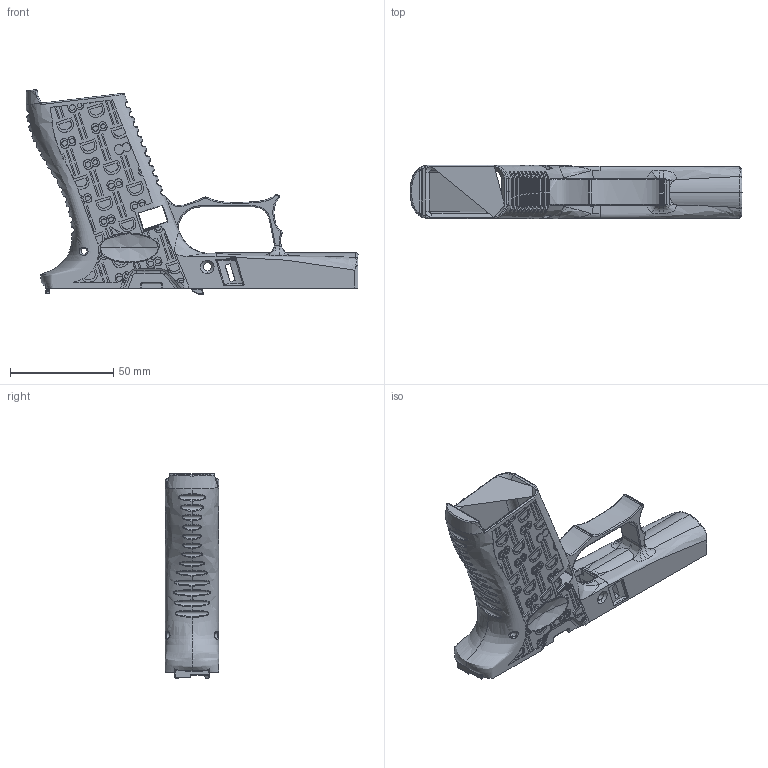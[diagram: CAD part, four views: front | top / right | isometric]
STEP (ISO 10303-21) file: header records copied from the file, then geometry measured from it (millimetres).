
FILE_DESCRIPTION (( 'STEP AP203' ), '1' );
FILE_NAME ('E43X DickinAround SLA.STEP', '2020-12-17T01:37:16', ( '' ), ( '' ), 'SwSTEP 2.0', 'SolidWorks 2016', '' );
FILE_SCHEMA (( 'CONFIG_CONTROL_DESIGN' ));
Products named in the file (1): E43X DickinAround SLA
Bounding box: 160.56 x 25.9 x 98.92 mm (x, y, z)
Volume: 61684.6 mm3; surface area: 39840.1 mm2
Topology: 1 solids, 1 shells, 2598 faces, 6892 edges, 4410 vertices
Faces by surface type: bspline 1189, plane 930, cylinder 433, torus 30, cone 12, sphere 4
Entity records: 383233 total; most frequent: CARTESIAN_POINT 329757, ORIENTED_EDGE 13674, EDGE_CURVE 6837, DIRECTION 6654, VERTEX_POINT 4410, B_SPLINE_CURVE_WITH_KNOTS 3459, EDGE_LOOP 2789, LINE 2686
